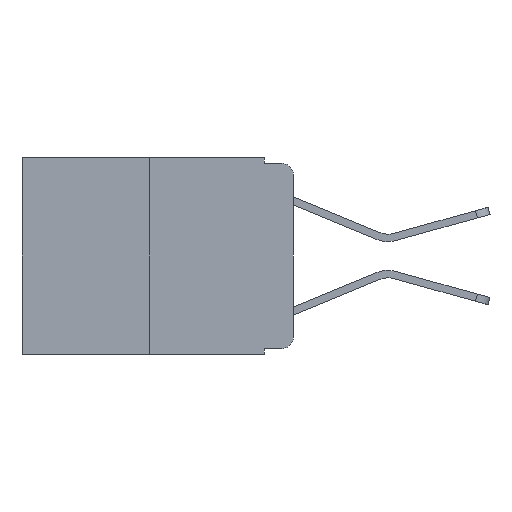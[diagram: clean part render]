
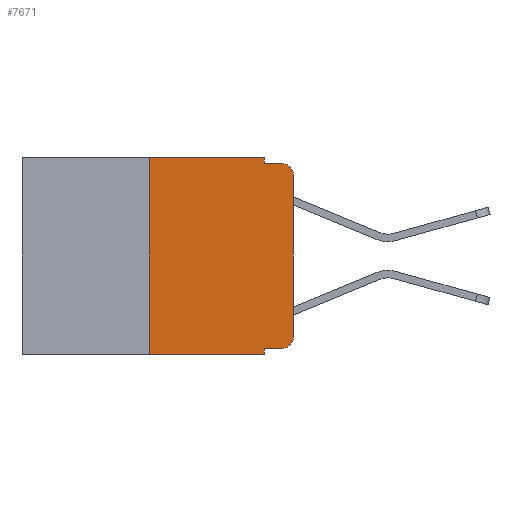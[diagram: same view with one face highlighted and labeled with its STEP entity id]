
A CAD part, left-side view. The second image highlights one B-rep face of the part: STEP entity #7671.
In plain terms, the highlighted planar face has unit normal (-1, 0, 0).
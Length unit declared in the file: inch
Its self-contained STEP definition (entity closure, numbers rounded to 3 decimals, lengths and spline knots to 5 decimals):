
#160 = ORIENTED_EDGE ( 'NONE', *, *, #6477, .F. ) ;
#166 = DIRECTION ( 'NONE',  ( -1., 0., 0. ) ) ;
#292 = CARTESIAN_POINT ( 'NONE',  ( 0., 0.473, 0. ) ) ;
#295 = ORIENTED_EDGE ( 'NONE', *, *, #4172, .T. ) ;
#382 = CARTESIAN_POINT ( 'NONE',  ( 0., 0.02, -0.03 ) ) ;
#518 = CARTESIAN_POINT ( 'NONE',  ( 0., 0.051, -0.01 ) ) ;
#522 = VECTOR ( 'NONE', #5825, 39.37008 ) ;
#543 = DIRECTION ( 'NONE',  ( 0., 0., -1. ) ) ;
#547 = FACE_OUTER_BOUND ( 'NONE', #9331, .T. ) ;
#564 = CARTESIAN_POINT ( 'NONE',  ( 0., 0., -0.313 ) ) ;
#568 = LINE ( 'NONE', #1221, #9857 ) ;
#571 = VECTOR ( 'NONE', #3182, 39.37008 ) ;
#698 = LINE ( 'NONE', #6275, #6116 ) ;
#1024 = ORIENTED_EDGE ( 'NONE', *, *, #6345, .T. ) ;
#1120 = VERTEX_POINT ( 'NONE', #564 ) ;
#1202 = LINE ( 'NONE', #292, #8298 ) ;
#1221 = CARTESIAN_POINT ( 'NONE',  ( 0., 0.051, 0. ) ) ;
#1222 = LINE ( 'NONE', #518, #8590 ) ;
#1248 = CARTESIAN_POINT ( 'NONE',  ( 0., 0.051, -0.333 ) ) ;
#1357 = ORIENTED_EDGE ( 'NONE', *, *, #2377, .F. ) ;
#1446 = CARTESIAN_POINT ( 'NONE',  ( 0., 0.02, -0.313 ) ) ;
#1592 = CARTESIAN_POINT ( 'NONE',  ( 0., 0.02, -0.01 ) ) ;
#2080 = DIRECTION ( 'NONE',  ( 0., 0., 1. ) ) ;
#2339 = CARTESIAN_POINT ( 'NONE',  ( 0., 0.051, -0.01 ) ) ;
#2377 = EDGE_CURVE ( 'NONE', #10217, #8498, #5344, .T. ) ;
#2750 = EDGE_CURVE ( 'NONE', #2856, #4123, #1222, .T. ) ;
#2782 = ORIENTED_EDGE ( 'NONE', *, *, #8399, .T. ) ;
#2856 = VERTEX_POINT ( 'NONE', #2339 ) ;
#2894 = CARTESIAN_POINT ( 'NONE',  ( 0., 0.25, 0. ) ) ;
#3067 = DIRECTION ( 'NONE',  ( 1., 0., 0. ) ) ;
#3182 = DIRECTION ( 'NONE',  ( 0., 0., -1. ) ) ;
#3561 = EDGE_CURVE ( 'NONE', #8498, #6515, #1202, .T. ) ;
#3677 = DIRECTION ( 'NONE',  ( 0., 0., -1. ) ) ;
#3692 = CIRCLE ( 'NONE', #9743, 0.02 ) ;
#3728 = CARTESIAN_POINT ( 'NONE',  ( 0., 0.473, 0. ) ) ;
#3934 = CARTESIAN_POINT ( 'NONE',  ( 0., 0.051, 0. ) ) ;
#4123 = VERTEX_POINT ( 'NONE', #1592 ) ;
#4172 = EDGE_CURVE ( 'NONE', #1120, #4950, #9866, .T. ) ;
#4300 = AXIS2_PLACEMENT_3D ( 'NONE', #1446, #166, #9932 ) ;
#4422 = VECTOR ( 'NONE', #2080, 39.37008 ) ;
#4630 = CARTESIAN_POINT ( 'NONE',  ( 0., 0.25, -0.343 ) ) ;
#4657 = ORIENTED_EDGE ( 'NONE', *, *, #7876, .T. ) ;
#4813 = LINE ( 'NONE', #3934, #571 ) ;
#4950 = VERTEX_POINT ( 'NONE', #9472 ) ;
#5344 = LINE ( 'NONE', #2894, #4422 ) ;
#5400 = DIRECTION ( 'NONE',  ( 0., -1., 0. ) ) ;
#5473 = EDGE_CURVE ( 'NONE', #6515, #2856, #568, .T. ) ;
#5580 = ORIENTED_EDGE ( 'NONE', *, *, #5473, .F. ) ;
#5784 = CARTESIAN_POINT ( 'NONE',  ( 0., 0.02, -0.333 ) ) ;
#5825 = DIRECTION ( 'NONE',  ( 0., 0., 1. ) ) ;
#5952 = CARTESIAN_POINT ( 'NONE',  ( 0., 0.473, -0.343 ) ) ;
#5968 = VECTOR ( 'NONE', #8335, 39.37008 ) ;
#6093 = DIRECTION ( 'NONE',  ( 0., 0., -1. ) ) ;
#6116 = VECTOR ( 'NONE', #5400, 39.37008 ) ;
#6119 = DIRECTION ( 'NONE',  ( -1., 0., 0. ) ) ;
#6175 = PLANE ( 'NONE',  #7351 ) ;
#6275 = CARTESIAN_POINT ( 'NONE',  ( 0., 0.051, -0.333 ) ) ;
#6345 = EDGE_CURVE ( 'NONE', #4950, #4123, #3692, .T. ) ;
#6357 = DIRECTION ( 'NONE',  ( 0., -1., 0. ) ) ;
#6386 = VERTEX_POINT ( 'NONE', #1248 ) ;
#6477 = EDGE_CURVE ( 'NONE', #6386, #8879, #4813, .T. ) ;
#6515 = VERTEX_POINT ( 'NONE', #7435 ) ;
#6912 = CIRCLE ( 'NONE', #4300, 0.02 ) ;
#7107 = DIRECTION ( 'NONE',  ( 0., -1., 0. ) ) ;
#7351 = AXIS2_PLACEMENT_3D ( 'NONE', #3728, #3067, #3677 ) ;
#7435 = CARTESIAN_POINT ( 'NONE',  ( 0., 0.051, 0. ) ) ;
#7516 = CARTESIAN_POINT ( 'NONE',  ( 0., 0., 0. ) ) ;
#7586 = CARTESIAN_POINT ( 'NONE',  ( 0., 0.25, 0. ) ) ;
#7671 = ADVANCED_FACE ( 'NONE', ( #547 ), #6175, .F. ) ;
#7726 = ORIENTED_EDGE ( 'NONE', *, *, #2750, .F. ) ;
#7876 = EDGE_CURVE ( 'NONE', #10217, #8879, #8384, .T. ) ;
#7898 = ORIENTED_EDGE ( 'NONE', *, *, #9830, .T. ) ;
#8270 = VERTEX_POINT ( 'NONE', #5784 ) ;
#8298 = VECTOR ( 'NONE', #7107, 39.37008 ) ;
#8335 = DIRECTION ( 'NONE',  ( 0., -1., 0. ) ) ;
#8384 = LINE ( 'NONE', #5952, #5968 ) ;
#8399 = EDGE_CURVE ( 'NONE', #8270, #1120, #6912, .T. ) ;
#8471 = CARTESIAN_POINT ( 'NONE',  ( 0., 0.051, -0.343 ) ) ;
#8498 = VERTEX_POINT ( 'NONE', #7586 ) ;
#8590 = VECTOR ( 'NONE', #6357, 39.37008 ) ;
#8879 = VERTEX_POINT ( 'NONE', #8471 ) ;
#9331 = EDGE_LOOP ( 'NONE', ( #295, #1024, #7726, #5580, #9860, #1357, #4657, #160, #7898, #2782 ) ) ;
#9472 = CARTESIAN_POINT ( 'NONE',  ( 0., 0., -0.03 ) ) ;
#9743 = AXIS2_PLACEMENT_3D ( 'NONE', #382, #6119, #543 ) ;
#9830 = EDGE_CURVE ( 'NONE', #6386, #8270, #698, .T. ) ;
#9857 = VECTOR ( 'NONE', #6093, 39.37008 ) ;
#9860 = ORIENTED_EDGE ( 'NONE', *, *, #3561, .F. ) ;
#9866 = LINE ( 'NONE', #7516, #522 ) ;
#9932 = DIRECTION ( 'NONE',  ( 0., 0., -1. ) ) ;
#10217 = VERTEX_POINT ( 'NONE', #4630 ) ;
